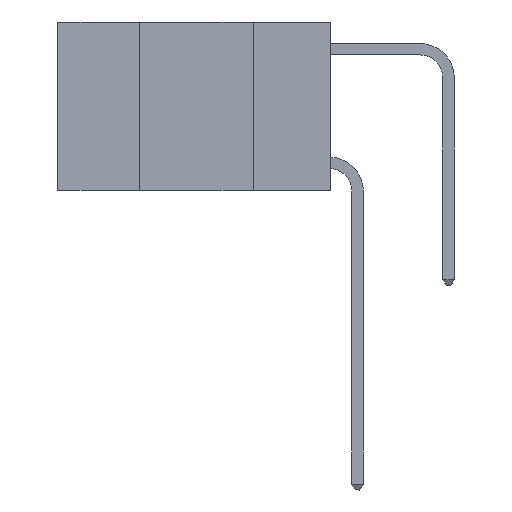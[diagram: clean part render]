
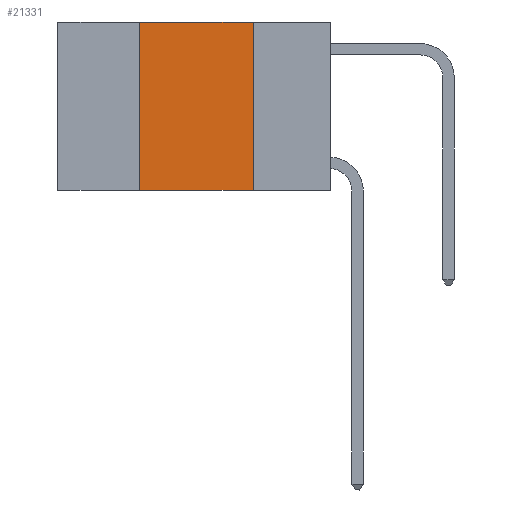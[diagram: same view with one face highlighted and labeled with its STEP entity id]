
A CAD part, left-side view. The second image highlights one B-rep face of the part: STEP entity #21331.
In plain terms, the highlighted planar face has unit normal (-1, 0, 0).
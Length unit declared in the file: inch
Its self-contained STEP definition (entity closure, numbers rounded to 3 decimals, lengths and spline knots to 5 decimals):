
#400 = EDGE_LOOP ( 'NONE', ( #13789, #14344, #836, #5540 ) ) ;
#416 = AXIS2_PLACEMENT_3D ( 'NONE', #2563, #6073, #18408 ) ;
#836 = ORIENTED_EDGE ( 'NONE', *, *, #13752, .F. ) ;
#1187 = CARTESIAN_POINT ( 'NONE',  ( 0., 0.6, -0.37 ) ) ;
#2563 = CARTESIAN_POINT ( 'NONE',  ( 0., 0.6, 0. ) ) ;
#4094 = CARTESIAN_POINT ( 'NONE',  ( 0., 0.17, 0. ) ) ;
#5540 = ORIENTED_EDGE ( 'NONE', *, *, #11388, .T. ) ;
#6073 = DIRECTION ( 'NONE',  ( 1., 0., 0. ) ) ;
#6381 = CARTESIAN_POINT ( 'NONE',  ( 0., 0.42, 0. ) ) ;
#6778 = CARTESIAN_POINT ( 'NONE',  ( 0., 0.42, -0.37 ) ) ;
#7680 = VECTOR ( 'NONE', #21675, 39.37008 ) ;
#7817 = EDGE_CURVE ( 'NONE', #16925, #19411, #15300, .T. ) ;
#7905 = CARTESIAN_POINT ( 'NONE',  ( 0., 0.42, 0. ) ) ;
#11120 = DIRECTION ( 'NONE',  ( 0., -1., 0. ) ) ;
#11388 = EDGE_CURVE ( 'NONE', #22409, #13366, #18567, .T. ) ;
#12355 = LINE ( 'NONE', #4094, #7680 ) ;
#13366 = VERTEX_POINT ( 'NONE', #15666 ) ;
#13752 = EDGE_CURVE ( 'NONE', #22409, #16925, #17366, .T. ) ;
#13789 = ORIENTED_EDGE ( 'NONE', *, *, #14930, .F. ) ;
#14344 = ORIENTED_EDGE ( 'NONE', *, *, #7817, .F. ) ;
#14930 = EDGE_CURVE ( 'NONE', #19411, #13366, #12355, .T. ) ;
#15276 = DIRECTION ( 'NONE',  ( 0., -1., 0. ) ) ;
#15300 = LINE ( 'NONE', #19874, #19416 ) ;
#15666 = CARTESIAN_POINT ( 'NONE',  ( 0., 0.17, -0.37 ) ) ;
#16682 = CARTESIAN_POINT ( 'NONE',  ( 0., 0.17, 0. ) ) ;
#16925 = VERTEX_POINT ( 'NONE', #6381 ) ;
#17366 = LINE ( 'NONE', #7905, #17922 ) ;
#17922 = VECTOR ( 'NONE', #20184, 39.37008 ) ;
#18339 = PLANE ( 'NONE',  #416 ) ;
#18408 = DIRECTION ( 'NONE',  ( 0., 0., -1. ) ) ;
#18567 = LINE ( 'NONE', #1187, #22638 ) ;
#19411 = VERTEX_POINT ( 'NONE', #16682 ) ;
#19416 = VECTOR ( 'NONE', #11120, 39.37008 ) ;
#19657 = FACE_OUTER_BOUND ( 'NONE', #400, .T. ) ;
#19874 = CARTESIAN_POINT ( 'NONE',  ( 0., 0.6, 0. ) ) ;
#20184 = DIRECTION ( 'NONE',  ( 0., 0., 1. ) ) ;
#21331 = ADVANCED_FACE ( 'NONE', ( #19657 ), #18339, .F. ) ;
#21675 = DIRECTION ( 'NONE',  ( 0., 0., -1. ) ) ;
#22409 = VERTEX_POINT ( 'NONE', #6778 ) ;
#22638 = VECTOR ( 'NONE', #15276, 39.37008 ) ;
